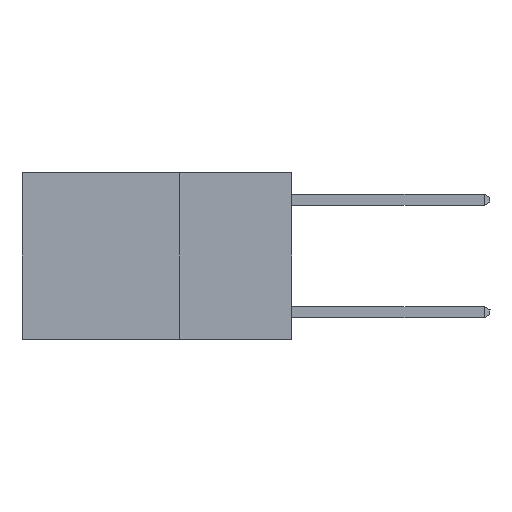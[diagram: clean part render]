
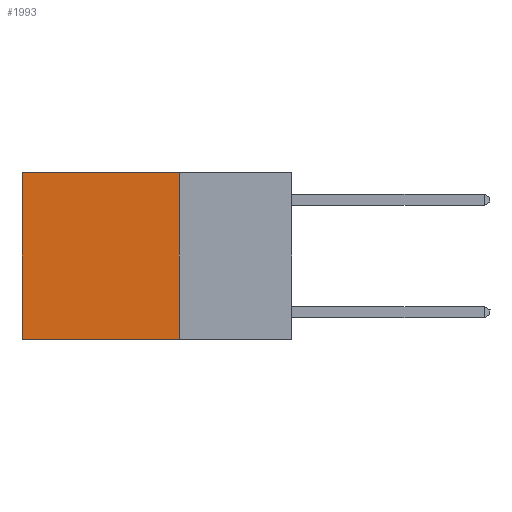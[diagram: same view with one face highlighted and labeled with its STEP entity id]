
A CAD part, left-side view. The second image highlights one B-rep face of the part: STEP entity #1993.
In plain terms, the highlighted planar face has unit normal (-1, 0, 0).
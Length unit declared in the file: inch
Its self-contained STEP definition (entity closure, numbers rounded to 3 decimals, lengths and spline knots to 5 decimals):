
#859 = LINE ( 'NONE', #14726, #15935 ) ;
#1857 = VECTOR ( 'NONE', #18632, 39.37008 ) ;
#1993 = ADVANCED_FACE ( 'NONE', ( #8425 ), #13787, .F. ) ;
#2199 = CARTESIAN_POINT ( 'NONE',  ( 0.2625, 0.6, 0. ) ) ;
#2590 = CARTESIAN_POINT ( 'NONE',  ( 0.2625, 0.25, 0. ) ) ;
#3289 = DIRECTION ( 'NONE',  ( 0., 1., 0. ) ) ;
#3935 = EDGE_CURVE ( 'NONE', #8329, #17763, #7759, .T. ) ;
#4219 = CARTESIAN_POINT ( 'NONE',  ( 0.2625, 0.25, 0. ) ) ;
#4290 = VECTOR ( 'NONE', #3289, 39.37008 ) ;
#5047 = EDGE_LOOP ( 'NONE', ( #7791, #7847, #7931, #8163 ) ) ;
#6416 = LINE ( 'NONE', #17281, #1857 ) ;
#6476 = LINE ( 'NONE', #2590, #13654 ) ;
#6633 = CARTESIAN_POINT ( 'NONE',  ( 0.2625, 0.25, -0.37 ) ) ;
#6661 = DIRECTION ( 'NONE',  ( 0., 0., -1. ) ) ;
#7022 = EDGE_CURVE ( 'NONE', #8329, #12153, #6476, .T. ) ;
#7759 = LINE ( 'NONE', #13489, #4290 ) ;
#7791 = ORIENTED_EDGE ( 'NONE', *, *, #16580, .T. ) ;
#7847 = ORIENTED_EDGE ( 'NONE', *, *, #11850, .F. ) ;
#7931 = ORIENTED_EDGE ( 'NONE', *, *, #7022, .F. ) ;
#8091 = CARTESIAN_POINT ( 'NONE',  ( 0.2625, 0.25, 0. ) ) ;
#8163 = ORIENTED_EDGE ( 'NONE', *, *, #3935, .T. ) ;
#8329 = VERTEX_POINT ( 'NONE', #4219 ) ;
#8425 = FACE_OUTER_BOUND ( 'NONE', #5047, .T. ) ;
#9258 = DIRECTION ( 'NONE',  ( 0., 0., -1. ) ) ;
#11524 = DIRECTION ( 'NONE',  ( 0., 0., -1. ) ) ;
#11850 = EDGE_CURVE ( 'NONE', #12153, #15976, #6416, .T. ) ;
#12105 = AXIS2_PLACEMENT_3D ( 'NONE', #8091, #15161, #6661 ) ;
#12153 = VERTEX_POINT ( 'NONE', #6633 ) ;
#13489 = CARTESIAN_POINT ( 'NONE',  ( 0.2625, 0.25, 0. ) ) ;
#13654 = VECTOR ( 'NONE', #11524, 39.37008 ) ;
#13787 = PLANE ( 'NONE',  #12105 ) ;
#14726 = CARTESIAN_POINT ( 'NONE',  ( 0.2625, 0.6, 0. ) ) ;
#15161 = DIRECTION ( 'NONE',  ( 1., 0., 0. ) ) ;
#15935 = VECTOR ( 'NONE', #9258, 39.37008 ) ;
#15976 = VERTEX_POINT ( 'NONE', #16651 ) ;
#16580 = EDGE_CURVE ( 'NONE', #17763, #15976, #859, .T. ) ;
#16651 = CARTESIAN_POINT ( 'NONE',  ( 0.2625, 0.6, -0.37 ) ) ;
#17281 = CARTESIAN_POINT ( 'NONE',  ( 0.2625, 0.25, -0.37 ) ) ;
#17763 = VERTEX_POINT ( 'NONE', #2199 ) ;
#18632 = DIRECTION ( 'NONE',  ( 0., 1., 0. ) ) ;
